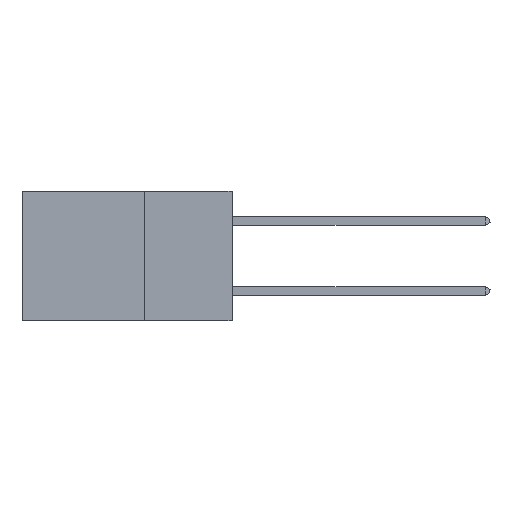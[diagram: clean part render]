
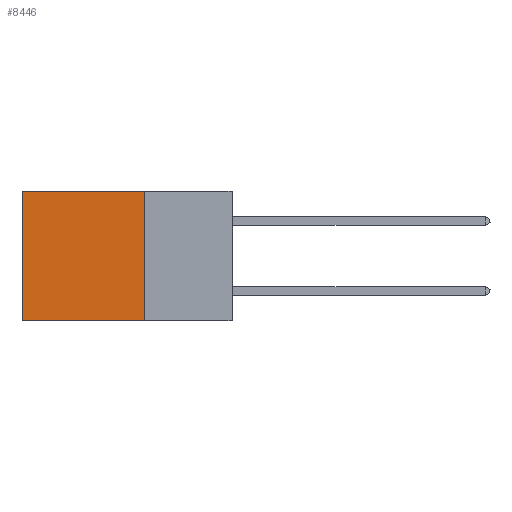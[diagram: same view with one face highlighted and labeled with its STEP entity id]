
A CAD part, left-side view. The second image highlights one B-rep face of the part: STEP entity #8446.
In plain terms, the highlighted planar face has unit normal (-1, 0, 0).
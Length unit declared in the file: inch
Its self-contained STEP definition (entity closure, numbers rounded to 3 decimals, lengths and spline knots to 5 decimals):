
#19 = ORIENTED_EDGE ( 'NONE', *, *, #29152, .T. ) ;
#393 = VECTOR ( 'NONE', #37735, 39.37008 ) ;
#462 = CARTESIAN_POINT ( 'NONE',  ( 0.2875, 0.6, 0. ) ) ;
#692 = DIRECTION ( 'NONE',  ( 0., 1., 0. ) ) ;
#4447 = DIRECTION ( 'NONE',  ( 0., 0., -1. ) ) ;
#6252 = CARTESIAN_POINT ( 'NONE',  ( 0.2875, 0.6, 0. ) ) ;
#7482 = CARTESIAN_POINT ( 'NONE',  ( 0.2875, 0.25, -0.37 ) ) ;
#8446 = ADVANCED_FACE ( 'NONE', ( #28853 ), #17737, .F. ) ;
#10063 = VERTEX_POINT ( 'NONE', #6252 ) ;
#10246 = CARTESIAN_POINT ( 'NONE',  ( 0.2875, 0.25, 0. ) ) ;
#10425 = LINE ( 'NONE', #7482, #393 ) ;
#11608 = EDGE_LOOP ( 'NONE', ( #19, #26142, #22379, #32248 ) ) ;
#12490 = VERTEX_POINT ( 'NONE', #40825 ) ;
#17737 = PLANE ( 'NONE',  #44856 ) ;
#18109 = VERTEX_POINT ( 'NONE', #32593 ) ;
#19285 = EDGE_CURVE ( 'NONE', #12490, #18109, #10425, .T. ) ;
#19369 = CARTESIAN_POINT ( 'NONE',  ( 0.2875, 0.25, 0. ) ) ;
#21465 = DIRECTION ( 'NONE',  ( 0., 0., -1. ) ) ;
#22379 = ORIENTED_EDGE ( 'NONE', *, *, #38914, .F. ) ;
#23972 = VECTOR ( 'NONE', #692, 39.37008 ) ;
#25356 = DIRECTION ( 'NONE',  ( 0., 0., -1. ) ) ;
#25667 = EDGE_CURVE ( 'NONE', #39152, #10063, #25714, .T. ) ;
#25714 = LINE ( 'NONE', #19369, #23972 ) ;
#26142 = ORIENTED_EDGE ( 'NONE', *, *, #19285, .F. ) ;
#26168 = LINE ( 'NONE', #45604, #29710 ) ;
#26278 = LINE ( 'NONE', #462, #45230 ) ;
#28853 = FACE_OUTER_BOUND ( 'NONE', #11608, .T. ) ;
#29152 = EDGE_CURVE ( 'NONE', #10063, #18109, #26278, .T. ) ;
#29710 = VECTOR ( 'NONE', #21465, 39.37008 ) ;
#32248 = ORIENTED_EDGE ( 'NONE', *, *, #25667, .T. ) ;
#32593 = CARTESIAN_POINT ( 'NONE',  ( 0.2875, 0.6, -0.37 ) ) ;
#36790 = DIRECTION ( 'NONE',  ( 1., 0., 0. ) ) ;
#37735 = DIRECTION ( 'NONE',  ( 0., 1., 0. ) ) ;
#38914 = EDGE_CURVE ( 'NONE', #39152, #12490, #26168, .T. ) ;
#39152 = VERTEX_POINT ( 'NONE', #10246 ) ;
#40825 = CARTESIAN_POINT ( 'NONE',  ( 0.2875, 0.25, -0.37 ) ) ;
#44557 = CARTESIAN_POINT ( 'NONE',  ( 0.2875, 0.25, 0. ) ) ;
#44856 = AXIS2_PLACEMENT_3D ( 'NONE', #44557, #36790, #25356 ) ;
#45230 = VECTOR ( 'NONE', #4447, 39.37008 ) ;
#45604 = CARTESIAN_POINT ( 'NONE',  ( 0.2875, 0.25, 0. ) ) ;
